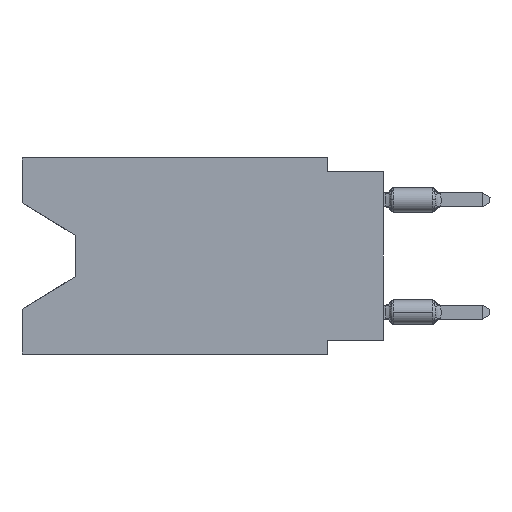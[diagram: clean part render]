
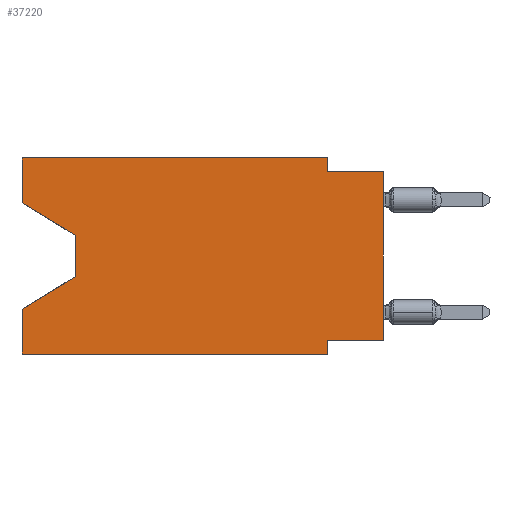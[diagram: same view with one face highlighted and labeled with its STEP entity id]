
A CAD part, left-side view. The second image highlights one B-rep face of the part: STEP entity #37220.
In plain terms, the highlighted planar face has unit normal (-1, 0, 0).
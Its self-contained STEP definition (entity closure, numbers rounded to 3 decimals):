
#298 = CARTESIAN_POINT ( 'NONE',  ( 0., 0., -8.255 ) ) ;
#506 = LINE ( 'NONE', #298, #20883 ) ;
#520 = VECTOR ( 'NONE', #1468, 1000. ) ;
#862 = LINE ( 'NONE', #3945, #12771 ) ;
#926 = VERTEX_POINT ( 'NONE', #14828 ) ;
#932 = CARTESIAN_POINT ( 'NONE',  ( 0., 16.383, -2.038 ) ) ;
#1036 = EDGE_CURVE ( 'NONE', #28962, #4287, #862, .T. ) ;
#1351 = LINE ( 'NONE', #24156, #14730 ) ;
#1468 = DIRECTION ( 'NONE',  ( 0., -0.855, -0.519 ) ) ;
#1915 = CARTESIAN_POINT ( 'NONE',  ( 0., 0., 0. ) ) ;
#2012 = EDGE_CURVE ( 'NONE', #24460, #4287, #16959, .T. ) ;
#2174 = VERTEX_POINT ( 'NONE', #32427 ) ;
#2587 = LINE ( 'NONE', #14362, #22973 ) ;
#2835 = ORIENTED_EDGE ( 'NONE', *, *, #3148, .F. ) ;
#2867 = ORIENTED_EDGE ( 'NONE', *, *, #22441, .F. ) ;
#3043 = DIRECTION ( 'NONE',  ( 0., 0., 1. ) ) ;
#3148 = EDGE_CURVE ( 'NONE', #17259, #27205, #1351, .T. ) ;
#3840 = EDGE_CURVE ( 'NONE', #13762, #23055, #36101, .T. ) ;
#3945 = CARTESIAN_POINT ( 'NONE',  ( 0., 0., -0.635 ) ) ;
#4287 = VERTEX_POINT ( 'NONE', #24056 ) ;
#5554 = DIRECTION ( 'NONE',  ( 0., -1., 0. ) ) ;
#6107 = DIRECTION ( 'NONE',  ( 0., 1., 0. ) ) ;
#6229 = VECTOR ( 'NONE', #8277, 1000. ) ;
#6451 = ORIENTED_EDGE ( 'NONE', *, *, #17563, .F. ) ;
#7072 = DIRECTION ( 'NONE',  ( 1., 0., 0. ) ) ;
#8077 = DIRECTION ( 'NONE',  ( 0., 0., -1. ) ) ;
#8277 = DIRECTION ( 'NONE',  ( 0., 0., 1. ) ) ;
#8706 = CARTESIAN_POINT ( 'NONE',  ( 0., 2.54, -8.255 ) ) ;
#8813 = CARTESIAN_POINT ( 'NONE',  ( 0., 16.383, -8.89 ) ) ;
#9013 = ORIENTED_EDGE ( 'NONE', *, *, #24144, .T. ) ;
#9208 = EDGE_CURVE ( 'NONE', #11827, #27205, #26215, .T. ) ;
#10324 = DIRECTION ( 'NONE',  ( 0., -1., 0. ) ) ;
#10637 = ORIENTED_EDGE ( 'NONE', *, *, #1036, .F. ) ;
#11312 = VECTOR ( 'NONE', #30745, 1000. ) ;
#11827 = VERTEX_POINT ( 'NONE', #27310 ) ;
#12499 = DIRECTION ( 'NONE',  ( 0., 0., -1. ) ) ;
#12771 = VECTOR ( 'NONE', #10324, 1000. ) ;
#12779 = EDGE_CURVE ( 'NONE', #2174, #37617, #2587, .T. ) ;
#12895 = CARTESIAN_POINT ( 'NONE',  ( 0., 16.383, 0. ) ) ;
#13062 = EDGE_LOOP ( 'NONE', ( #18513, #9013, #25716, #6451, #35003, #2835, #25396, #17005, #10637, #34168, #2867, #15944 ) ) ;
#13459 = DIRECTION ( 'NONE',  ( 0., -1., 0. ) ) ;
#13468 = AXIS2_PLACEMENT_3D ( 'NONE', #12895, #7072, #12499 ) ;
#13762 = VERTEX_POINT ( 'NONE', #932 ) ;
#13785 = VECTOR ( 'NONE', #13459, 1000. ) ;
#14075 = DIRECTION ( 'NONE',  ( 0., 0., 1. ) ) ;
#14271 = CARTESIAN_POINT ( 'NONE',  ( 0., 16.383, 0. ) ) ;
#14362 = CARTESIAN_POINT ( 'NONE',  ( 0., 13.97, -5.385 ) ) ;
#14730 = VECTOR ( 'NONE', #35967, 1000. ) ;
#14828 = CARTESIAN_POINT ( 'NONE',  ( 0., 2.54, 0. ) ) ;
#15577 = LINE ( 'NONE', #24849, #13785 ) ;
#15944 = ORIENTED_EDGE ( 'NONE', *, *, #3840, .F. ) ;
#16959 = LINE ( 'NONE', #1915, #30749 ) ;
#17005 = ORIENTED_EDGE ( 'NONE', *, *, #2012, .T. ) ;
#17259 = VERTEX_POINT ( 'NONE', #8706 ) ;
#17563 = EDGE_CURVE ( 'NONE', #11827, #37617, #31506, .T. ) ;
#17838 = CARTESIAN_POINT ( 'NONE',  ( 0., 2.54, 0. ) ) ;
#18385 = CARTESIAN_POINT ( 'NONE',  ( 0., 16.383, 0. ) ) ;
#18513 = ORIENTED_EDGE ( 'NONE', *, *, #32250, .T. ) ;
#20883 = VECTOR ( 'NONE', #6107, 1000. ) ;
#21190 = CARTESIAN_POINT ( 'NONE',  ( 0., 16.383, 0. ) ) ;
#21383 = PLANE ( 'NONE',  #13468 ) ;
#22441 = EDGE_CURVE ( 'NONE', #23055, #926, #15577, .T. ) ;
#22692 = DIRECTION ( 'NONE',  ( 0., 0.855, -0.519 ) ) ;
#22776 = CARTESIAN_POINT ( 'NONE',  ( 0., 13.97, -3.505 ) ) ;
#22973 = VECTOR ( 'NONE', #22692, 1000. ) ;
#23055 = VERTEX_POINT ( 'NONE', #18385 ) ;
#23936 = VERTEX_POINT ( 'NONE', #34390 ) ;
#24056 = CARTESIAN_POINT ( 'NONE',  ( 0., 0., -0.635 ) ) ;
#24144 = EDGE_CURVE ( 'NONE', #23936, #2174, #35340, .T. ) ;
#24156 = CARTESIAN_POINT ( 'NONE',  ( 0., 2.54, -8.89 ) ) ;
#24460 = VERTEX_POINT ( 'NONE', #29057 ) ;
#24849 = CARTESIAN_POINT ( 'NONE',  ( 0., 16.383, 0. ) ) ;
#25396 = ORIENTED_EDGE ( 'NONE', *, *, #25788, .F. ) ;
#25716 = ORIENTED_EDGE ( 'NONE', *, *, #12779, .T. ) ;
#25788 = EDGE_CURVE ( 'NONE', #24460, #17259, #506, .T. ) ;
#25969 = CARTESIAN_POINT ( 'NONE',  ( 0., 2.54, -8.89 ) ) ;
#26168 = EDGE_CURVE ( 'NONE', #926, #28962, #27647, .T. ) ;
#26215 = LINE ( 'NONE', #8813, #30111 ) ;
#27205 = VERTEX_POINT ( 'NONE', #25969 ) ;
#27310 = CARTESIAN_POINT ( 'NONE',  ( 0., 16.383, -8.89 ) ) ;
#27647 = LINE ( 'NONE', #17838, #11312 ) ;
#28962 = VERTEX_POINT ( 'NONE', #35650 ) ;
#29057 = CARTESIAN_POINT ( 'NONE',  ( 0., 0., -8.255 ) ) ;
#30111 = VECTOR ( 'NONE', #5554, 1000. ) ;
#30459 = CARTESIAN_POINT ( 'NONE',  ( 0., 16.383, -2.038 ) ) ;
#30745 = DIRECTION ( 'NONE',  ( 0., 0., -1. ) ) ;
#30749 = VECTOR ( 'NONE', #14075, 1000. ) ;
#31506 = LINE ( 'NONE', #14271, #6229 ) ;
#32250 = EDGE_CURVE ( 'NONE', #13762, #23936, #36083, .T. ) ;
#32427 = CARTESIAN_POINT ( 'NONE',  ( 0., 13.97, -5.385 ) ) ;
#33308 = VECTOR ( 'NONE', #3043, 1000. ) ;
#33344 = CARTESIAN_POINT ( 'NONE',  ( 0., 16.383, -6.852 ) ) ;
#33772 = FACE_OUTER_BOUND ( 'NONE', #13062, .T. ) ;
#34168 = ORIENTED_EDGE ( 'NONE', *, *, #26168, .F. ) ;
#34390 = CARTESIAN_POINT ( 'NONE',  ( 0., 13.97, -3.505 ) ) ;
#35003 = ORIENTED_EDGE ( 'NONE', *, *, #9208, .T. ) ;
#35340 = LINE ( 'NONE', #22776, #36873 ) ;
#35650 = CARTESIAN_POINT ( 'NONE',  ( 0., 2.54, -0.635 ) ) ;
#35967 = DIRECTION ( 'NONE',  ( 0., 0., -1. ) ) ;
#36083 = LINE ( 'NONE', #30459, #520 ) ;
#36101 = LINE ( 'NONE', #21190, #33308 ) ;
#36873 = VECTOR ( 'NONE', #8077, 1000. ) ;
#37220 = ADVANCED_FACE ( 'NONE', ( #33772 ), #21383, .F. ) ;
#37617 = VERTEX_POINT ( 'NONE', #33344 ) ;
